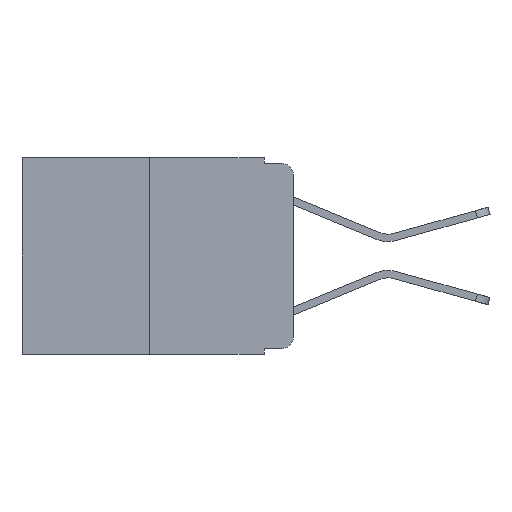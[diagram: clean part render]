
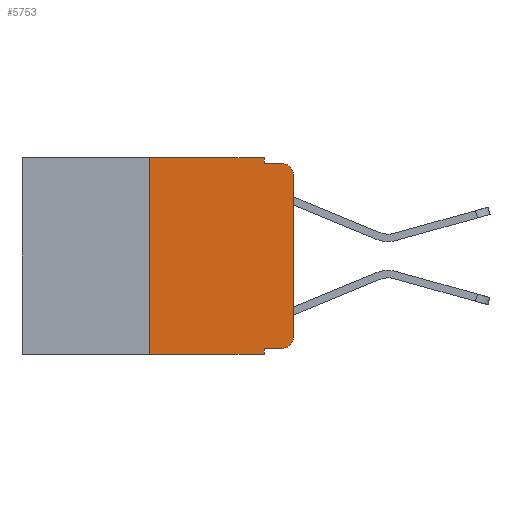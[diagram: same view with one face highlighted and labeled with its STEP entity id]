
A CAD part, left-side view. The second image highlights one B-rep face of the part: STEP entity #5753.
In plain terms, the highlighted planar face has unit normal (-1, 0, 0).
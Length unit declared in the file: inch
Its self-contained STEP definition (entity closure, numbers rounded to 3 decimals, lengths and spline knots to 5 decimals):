
#468 = AXIS2_PLACEMENT_3D ( 'NONE', #8147, #20567, #9914 ) ;
#497 = VECTOR ( 'NONE', #9468, 39.37008 ) ;
#572 = ORIENTED_EDGE ( 'NONE', *, *, #22932, .T. ) ;
#722 = VECTOR ( 'NONE', #18679, 39.37008 ) ;
#1024 = VERTEX_POINT ( 'NONE', #14791 ) ;
#1039 = VERTEX_POINT ( 'NONE', #13086 ) ;
#1103 = LINE ( 'NONE', #2154, #497 ) ;
#1116 = ORIENTED_EDGE ( 'NONE', *, *, #3334, .F. ) ;
#1470 = DIRECTION ( 'NONE',  ( -1., 0., 0. ) ) ;
#2154 = CARTESIAN_POINT ( 'NONE',  ( 0., 0.473, -0.343 ) ) ;
#2618 = VERTEX_POINT ( 'NONE', #11532 ) ;
#3334 = EDGE_CURVE ( 'NONE', #5006, #16369, #21825, .T. ) ;
#4371 = VECTOR ( 'NONE', #9135, 39.37008 ) ;
#4435 = CARTESIAN_POINT ( 'NONE',  ( 0., 0., -0.03 ) ) ;
#4465 = PLANE ( 'NONE',  #468 ) ;
#4520 = CARTESIAN_POINT ( 'NONE',  ( 0., 0.051, 0. ) ) ;
#4602 = EDGE_CURVE ( 'NONE', #1039, #13823, #23101, .T. ) ;
#4651 = DIRECTION ( 'NONE',  ( 0., 0., -1. ) ) ;
#4758 = CARTESIAN_POINT ( 'NONE',  ( 0., 0.051, -0.343 ) ) ;
#5006 = VERTEX_POINT ( 'NONE', #15107 ) ;
#5044 = DIRECTION ( 'NONE',  ( -1., 0., 0. ) ) ;
#5088 = DIRECTION ( 'NONE',  ( 0., 0., 1. ) ) ;
#5511 = CARTESIAN_POINT ( 'NONE',  ( 0., 0.473, 0. ) ) ;
#5753 = ADVANCED_FACE ( 'NONE', ( #14517 ), #4465, .F. ) ;
#5826 = ORIENTED_EDGE ( 'NONE', *, *, #7108, .F. ) ;
#5945 = ORIENTED_EDGE ( 'NONE', *, *, #21776, .T. ) ;
#6434 = VERTEX_POINT ( 'NONE', #16780 ) ;
#7108 = EDGE_CURVE ( 'NONE', #11811, #19031, #11798, .T. ) ;
#7937 = AXIS2_PLACEMENT_3D ( 'NONE', #15766, #5044, #17557 ) ;
#8147 = CARTESIAN_POINT ( 'NONE',  ( 0., 0.473, 0. ) ) ;
#8739 = EDGE_CURVE ( 'NONE', #13823, #11811, #18668, .T. ) ;
#8760 = LINE ( 'NONE', #19139, #21261 ) ;
#9042 = CIRCLE ( 'NONE', #7937, 0.02 ) ;
#9135 = DIRECTION ( 'NONE',  ( 0., -1., 0. ) ) ;
#9468 = DIRECTION ( 'NONE',  ( 0., -1., 0. ) ) ;
#9914 = DIRECTION ( 'NONE',  ( 0., 0., -1. ) ) ;
#10297 = ORIENTED_EDGE ( 'NONE', *, *, #13034, .T. ) ;
#10433 = CARTESIAN_POINT ( 'NONE',  ( 0., 0.051, -0.01 ) ) ;
#10644 = EDGE_CURVE ( 'NONE', #19031, #6434, #19952, .T. ) ;
#10729 = EDGE_LOOP ( 'NONE', ( #10297, #18640, #21923, #5826, #18106, #23026, #17010, #1116, #572, #5945 ) ) ;
#11350 = CIRCLE ( 'NONE', #23309, 0.02 ) ;
#11532 = CARTESIAN_POINT ( 'NONE',  ( 0., 0.02, -0.333 ) ) ;
#11664 = CARTESIAN_POINT ( 'NONE',  ( 0., 0.051, -0.01 ) ) ;
#11798 = LINE ( 'NONE', #4520, #21756 ) ;
#11811 = VERTEX_POINT ( 'NONE', #13812 ) ;
#11857 = EDGE_CURVE ( 'NONE', #14341, #6434, #9042, .T. ) ;
#11884 = CARTESIAN_POINT ( 'NONE',  ( 0., 0.25, 0. ) ) ;
#12410 = CARTESIAN_POINT ( 'NONE',  ( 0., 0.02, -0.313 ) ) ;
#13034 = EDGE_CURVE ( 'NONE', #1024, #14341, #14703, .T. ) ;
#13086 = CARTESIAN_POINT ( 'NONE',  ( 0., 0.25, -0.343 ) ) ;
#13812 = CARTESIAN_POINT ( 'NONE',  ( 0., 0.051, 0. ) ) ;
#13823 = VERTEX_POINT ( 'NONE', #11884 ) ;
#14011 = DIRECTION ( 'NONE',  ( 0., -1., 0. ) ) ;
#14194 = DIRECTION ( 'NONE',  ( 0., 0., -1. ) ) ;
#14341 = VERTEX_POINT ( 'NONE', #4435 ) ;
#14517 = FACE_OUTER_BOUND ( 'NONE', #10729, .T. ) ;
#14703 = LINE ( 'NONE', #20451, #722 ) ;
#14791 = CARTESIAN_POINT ( 'NONE',  ( 0., 0., -0.313 ) ) ;
#15107 = CARTESIAN_POINT ( 'NONE',  ( 0., 0.051, -0.333 ) ) ;
#15244 = VECTOR ( 'NONE', #14011, 39.37008 ) ;
#15766 = CARTESIAN_POINT ( 'NONE',  ( 0., 0.02, -0.03 ) ) ;
#16369 = VERTEX_POINT ( 'NONE', #4758 ) ;
#16780 = CARTESIAN_POINT ( 'NONE',  ( 0., 0.02, -0.01 ) ) ;
#17010 = ORIENTED_EDGE ( 'NONE', *, *, #18866, .T. ) ;
#17067 = DIRECTION ( 'NONE',  ( 0., 0., -1. ) ) ;
#17154 = VECTOR ( 'NONE', #4651, 39.37008 ) ;
#17337 = CARTESIAN_POINT ( 'NONE',  ( 0., 0.051, 0. ) ) ;
#17557 = DIRECTION ( 'NONE',  ( 0., 0., -1. ) ) ;
#18106 = ORIENTED_EDGE ( 'NONE', *, *, #8739, .F. ) ;
#18640 = ORIENTED_EDGE ( 'NONE', *, *, #11857, .T. ) ;
#18668 = LINE ( 'NONE', #5511, #4371 ) ;
#18679 = DIRECTION ( 'NONE',  ( 0., 0., 1. ) ) ;
#18866 = EDGE_CURVE ( 'NONE', #1039, #16369, #1103, .T. ) ;
#19026 = VECTOR ( 'NONE', #5088, 39.37008 ) ;
#19031 = VERTEX_POINT ( 'NONE', #11664 ) ;
#19139 = CARTESIAN_POINT ( 'NONE',  ( 0., 0.051, -0.333 ) ) ;
#19952 = LINE ( 'NONE', #10433, #15244 ) ;
#20451 = CARTESIAN_POINT ( 'NONE',  ( 0., 0., 0. ) ) ;
#20567 = DIRECTION ( 'NONE',  ( 1., 0., 0. ) ) ;
#20908 = DIRECTION ( 'NONE',  ( 0., -1., 0. ) ) ;
#21261 = VECTOR ( 'NONE', #20908, 39.37008 ) ;
#21756 = VECTOR ( 'NONE', #17067, 39.37008 ) ;
#21776 = EDGE_CURVE ( 'NONE', #2618, #1024, #11350, .T. ) ;
#21825 = LINE ( 'NONE', #17337, #17154 ) ;
#21923 = ORIENTED_EDGE ( 'NONE', *, *, #10644, .F. ) ;
#22801 = CARTESIAN_POINT ( 'NONE',  ( 0., 0.25, 0. ) ) ;
#22932 = EDGE_CURVE ( 'NONE', #5006, #2618, #8760, .T. ) ;
#23026 = ORIENTED_EDGE ( 'NONE', *, *, #4602, .F. ) ;
#23101 = LINE ( 'NONE', #22801, #19026 ) ;
#23309 = AXIS2_PLACEMENT_3D ( 'NONE', #12410, #1470, #14194 ) ;
